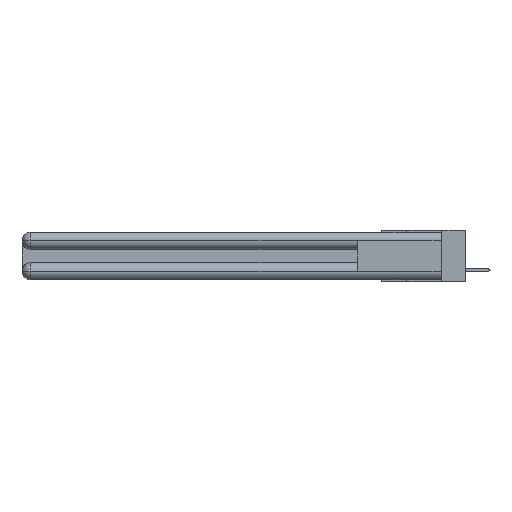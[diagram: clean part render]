
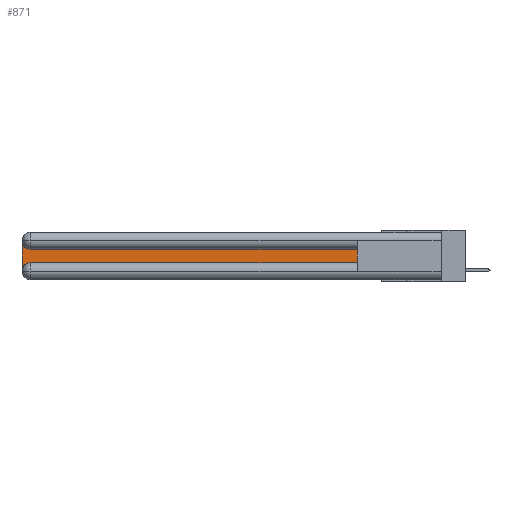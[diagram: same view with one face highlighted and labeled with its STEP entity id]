
A CAD part, left-side view. The second image highlights one B-rep face of the part: STEP entity #871.
In plain terms, the highlighted planar face has unit normal (-1, 0, 0).
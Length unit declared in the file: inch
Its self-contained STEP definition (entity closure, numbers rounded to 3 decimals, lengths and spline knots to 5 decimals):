
#270 = DIRECTION ( 'NONE',  ( 1., 0., 0. ) ) ;
#621 = DIRECTION ( 'NONE',  ( 0., 0., -1. ) ) ;
#862 = CIRCLE ( 'NONE', #15258, 0.06 ) ;
#871 = ADVANCED_FACE ( 'NONE', ( #1613 ), #2555, .F. ) ;
#1551 = LINE ( 'NONE', #26982, #27746 ) ;
#1613 = FACE_OUTER_BOUND ( 'NONE', #27070, .T. ) ;
#2046 = DIRECTION ( 'NONE',  ( 0., 1., 0. ) ) ;
#2515 = CARTESIAN_POINT ( 'NONE',  ( 0.075, 0.6, -0.1225 ) ) ;
#2555 = PLANE ( 'NONE',  #7717 ) ;
#2735 = CARTESIAN_POINT ( 'NONE',  ( 0.075, 3., -0.2175 ) ) ;
#4149 = VERTEX_POINT ( 'NONE', #23460 ) ;
#4770 = CARTESIAN_POINT ( 'NONE',  ( 0.075, 3., -0.1225 ) ) ;
#4944 = DIRECTION ( 'NONE',  ( 0., 0., 1. ) ) ;
#5124 = AXIS2_PLACEMENT_3D ( 'NONE', #22829, #14070, #23215 ) ;
#5492 = EDGE_CURVE ( 'NONE', #4149, #26292, #1551, .T. ) ;
#5851 = VECTOR ( 'NONE', #4944, 39.37008 ) ;
#7717 = AXIS2_PLACEMENT_3D ( 'NONE', #4770, #270, #17971 ) ;
#9253 = LINE ( 'NONE', #21473, #28234 ) ;
#10483 = CARTESIAN_POINT ( 'NONE',  ( 0.075, 2.94, -0.0625 ) ) ;
#10627 = EDGE_CURVE ( 'NONE', #14428, #27616, #21597, .T. ) ;
#11559 = ORIENTED_EDGE ( 'NONE', *, *, #16485, .T. ) ;
#11727 = LINE ( 'NONE', #19889, #5851 ) ;
#14070 = DIRECTION ( 'NONE',  ( 1., 0., 0. ) ) ;
#14428 = VERTEX_POINT ( 'NONE', #26273 ) ;
#14819 = ORIENTED_EDGE ( 'NONE', *, *, #17366, .T. ) ;
#15258 = AXIS2_PLACEMENT_3D ( 'NONE', #10483, #21475, #23812 ) ;
#15587 = CARTESIAN_POINT ( 'NONE',  ( 0.075, 2.94, -0.1225 ) ) ;
#15904 = DIRECTION ( 'NONE',  ( 0., -1., 0. ) ) ;
#16485 = EDGE_CURVE ( 'NONE', #26292, #24650, #11727, .T. ) ;
#17255 = CARTESIAN_POINT ( 'NONE',  ( 0.075, 3., -0.2775 ) ) ;
#17366 = EDGE_CURVE ( 'NONE', #27616, #4149, #18355, .T. ) ;
#17826 = VECTOR ( 'NONE', #621, 39.37008 ) ;
#17971 = DIRECTION ( 'NONE',  ( 0., 0., -1. ) ) ;
#18355 = CIRCLE ( 'NONE', #5124, 0.06 ) ;
#18627 = ORIENTED_EDGE ( 'NONE', *, *, #24406, .T. ) ;
#19889 = CARTESIAN_POINT ( 'NONE',  ( 0.075, 0.6, -0.2175 ) ) ;
#20725 = VERTEX_POINT ( 'NONE', #15587 ) ;
#21027 = ORIENTED_EDGE ( 'NONE', *, *, #10627, .T. ) ;
#21380 = CARTESIAN_POINT ( 'NONE',  ( 0.075, 0.6, -0.2175 ) ) ;
#21473 = CARTESIAN_POINT ( 'NONE',  ( 0.075, 0.6, -0.1225 ) ) ;
#21475 = DIRECTION ( 'NONE',  ( 1., 0., 0. ) ) ;
#21597 = LINE ( 'NONE', #2735, #17826 ) ;
#22538 = ORIENTED_EDGE ( 'NONE', *, *, #27475, .T. ) ;
#22829 = CARTESIAN_POINT ( 'NONE',  ( 0.075, 2.94, -0.2775 ) ) ;
#23215 = DIRECTION ( 'NONE',  ( 0., 0., -1. ) ) ;
#23460 = CARTESIAN_POINT ( 'NONE',  ( 0.075, 2.94, -0.2175 ) ) ;
#23812 = DIRECTION ( 'NONE',  ( 0., 0., -1. ) ) ;
#24406 = EDGE_CURVE ( 'NONE', #24650, #20725, #9253, .T. ) ;
#24650 = VERTEX_POINT ( 'NONE', #2515 ) ;
#25018 = ORIENTED_EDGE ( 'NONE', *, *, #5492, .T. ) ;
#26273 = CARTESIAN_POINT ( 'NONE',  ( 0.075, 3., -0.0625 ) ) ;
#26292 = VERTEX_POINT ( 'NONE', #21380 ) ;
#26982 = CARTESIAN_POINT ( 'NONE',  ( 0.075, 0.6, -0.2175 ) ) ;
#27070 = EDGE_LOOP ( 'NONE', ( #18627, #22538, #21027, #14819, #25018, #11559 ) ) ;
#27475 = EDGE_CURVE ( 'NONE', #20725, #14428, #862, .T. ) ;
#27616 = VERTEX_POINT ( 'NONE', #17255 ) ;
#27746 = VECTOR ( 'NONE', #15904, 39.37008 ) ;
#28234 = VECTOR ( 'NONE', #2046, 39.37008 ) ;
